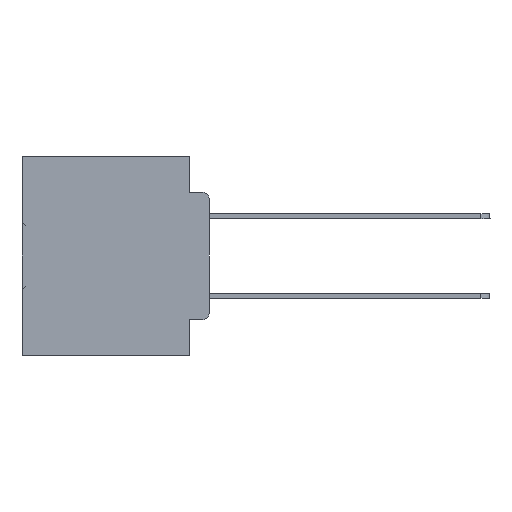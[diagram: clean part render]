
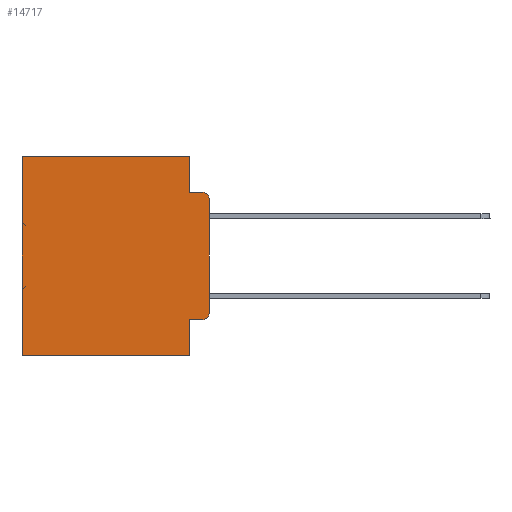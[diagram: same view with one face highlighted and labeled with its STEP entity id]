
A CAD part, left-side view. The second image highlights one B-rep face of the part: STEP entity #14717.
In plain terms, the highlighted planar face has unit normal (-1, 0, 0).
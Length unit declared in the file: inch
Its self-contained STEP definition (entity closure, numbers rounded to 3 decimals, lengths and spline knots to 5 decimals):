
#862 = CARTESIAN_POINT ( 'NONE',  ( 0.298, 0.051, 0. ) ) ;
#1146 = ORIENTED_EDGE ( 'NONE', *, *, #27035, .T. ) ;
#1176 = VERTEX_POINT ( 'NONE', #15526 ) ;
#2767 = DIRECTION ( 'NONE',  ( 0., 1., 0. ) ) ;
#3142 = DIRECTION ( 'NONE',  ( 0., 0., -1. ) ) ;
#3258 = LINE ( 'NONE', #32283, #28905 ) ;
#3944 = DIRECTION ( 'NONE',  ( 0., 1., 0. ) ) ;
#4277 = LINE ( 'NONE', #5706, #37632 ) ;
#4386 = VERTEX_POINT ( 'NONE', #31850 ) ;
#4535 = PLANE ( 'NONE',  #34466 ) ;
#4669 = CARTESIAN_POINT ( 'NONE',  ( 0.298, 0., 0. ) ) ;
#5588 = CARTESIAN_POINT ( 'NONE',  ( 0.298, 0., -0.3915 ) ) ;
#5706 = CARTESIAN_POINT ( 'NONE',  ( 0.298, 0., 0. ) ) ;
#5940 = DIRECTION ( 'NONE',  ( 0., -1., 0. ) ) ;
#7246 = DIRECTION ( 'NONE',  ( 1., 0., 0. ) ) ;
#7446 = VECTOR ( 'NONE', #3944, 39.37008 ) ;
#7640 = DIRECTION ( 'NONE',  ( 0., 0., -1. ) ) ;
#7863 = VERTEX_POINT ( 'NONE', #32480 ) ;
#8265 = DIRECTION ( 'NONE',  ( 0., 0., -1. ) ) ;
#9531 = EDGE_CURVE ( 'NONE', #37716, #35159, #14981, .T. ) ;
#9601 = EDGE_LOOP ( 'NONE', ( #37033, #34493, #10589, #10819, #17951, #32750, #32265, #28895, #12458, #1146 ) ) ;
#10589 = ORIENTED_EDGE ( 'NONE', *, *, #26523, .F. ) ;
#10819 = ORIENTED_EDGE ( 'NONE', *, *, #9531, .F. ) ;
#10880 = AXIS2_PLACEMENT_3D ( 'NONE', #23464, #20653, #3142 ) ;
#11862 = CARTESIAN_POINT ( 'NONE',  ( 0.298, 0.051, -0.0885 ) ) ;
#12153 = EDGE_CURVE ( 'NONE', #37716, #7863, #3258, .T. ) ;
#12458 = ORIENTED_EDGE ( 'NONE', *, *, #17534, .T. ) ;
#12671 = FACE_OUTER_BOUND ( 'NONE', #9601, .T. ) ;
#13833 = VECTOR ( 'NONE', #5940, 39.37008 ) ;
#14717 = ADVANCED_FACE ( 'NONE', ( #12671 ), #4535, .F. ) ;
#14981 = LINE ( 'NONE', #25881, #30955 ) ;
#15052 = CARTESIAN_POINT ( 'NONE',  ( 0.298, 0.051, -0.0885 ) ) ;
#15442 = EDGE_CURVE ( 'NONE', #1176, #4386, #32273, .T. ) ;
#15526 = CARTESIAN_POINT ( 'NONE',  ( 0.298, 0., -0.1085 ) ) ;
#15543 = CIRCLE ( 'NONE', #10880, 0.02 ) ;
#17014 = EDGE_CURVE ( 'NONE', #19408, #22976, #26633, .T. ) ;
#17534 = EDGE_CURVE ( 'NONE', #34117, #25563, #30653, .T. ) ;
#17951 = ORIENTED_EDGE ( 'NONE', *, *, #12153, .T. ) ;
#18342 = EDGE_CURVE ( 'NONE', #34117, #19408, #34751, .T. ) ;
#18680 = VERTEX_POINT ( 'NONE', #5588 ) ;
#18697 = DIRECTION ( 'NONE',  ( 0., 0., -1. ) ) ;
#19233 = CARTESIAN_POINT ( 'NONE',  ( 0.298, 0.051, -0.4115 ) ) ;
#19408 = VERTEX_POINT ( 'NONE', #31348 ) ;
#20653 = DIRECTION ( 'NONE',  ( -1., 0., 0. ) ) ;
#21307 = CARTESIAN_POINT ( 'NONE',  ( 0.298, 0., -0.5 ) ) ;
#21585 = CARTESIAN_POINT ( 'NONE',  ( 0.298, 0.051, -0.4115 ) ) ;
#22516 = LINE ( 'NONE', #31189, #34857 ) ;
#22976 = VERTEX_POINT ( 'NONE', #28055 ) ;
#23464 = CARTESIAN_POINT ( 'NONE',  ( 0.298, 0.02, -0.3915 ) ) ;
#25390 = DIRECTION ( 'NONE',  ( 0., -1., 0. ) ) ;
#25563 = VERTEX_POINT ( 'NONE', #34015 ) ;
#25881 = CARTESIAN_POINT ( 'NONE',  ( 0.298, 0.051, 0. ) ) ;
#26145 = VECTOR ( 'NONE', #25390, 39.37008 ) ;
#26523 = EDGE_CURVE ( 'NONE', #35159, #4386, #37072, .T. ) ;
#26633 = LINE ( 'NONE', #21307, #7446 ) ;
#27035 = EDGE_CURVE ( 'NONE', #25563, #18680, #15543, .T. ) ;
#27625 = AXIS2_PLACEMENT_3D ( 'NONE', #33479, #33345, #36796 ) ;
#28055 = CARTESIAN_POINT ( 'NONE',  ( 0.298, 0.473, -0.5 ) ) ;
#28895 = ORIENTED_EDGE ( 'NONE', *, *, #18342, .F. ) ;
#28905 = VECTOR ( 'NONE', #2767, 39.37008 ) ;
#29671 = VECTOR ( 'NONE', #18697, 39.37008 ) ;
#29848 = DIRECTION ( 'NONE',  ( 0., 0., -1. ) ) ;
#30209 = EDGE_CURVE ( 'NONE', #7863, #22976, #22516, .T. ) ;
#30653 = LINE ( 'NONE', #19233, #26145 ) ;
#30955 = VECTOR ( 'NONE', #8265, 39.37008 ) ;
#31189 = CARTESIAN_POINT ( 'NONE',  ( 0.298, 0.473, 0. ) ) ;
#31348 = CARTESIAN_POINT ( 'NONE',  ( 0.298, 0.051, -0.5 ) ) ;
#31850 = CARTESIAN_POINT ( 'NONE',  ( 0.298, 0.02, -0.0885 ) ) ;
#32265 = ORIENTED_EDGE ( 'NONE', *, *, #17014, .F. ) ;
#32273 = CIRCLE ( 'NONE', #27625, 0.02 ) ;
#32283 = CARTESIAN_POINT ( 'NONE',  ( 0.298, 0., 0. ) ) ;
#32480 = CARTESIAN_POINT ( 'NONE',  ( 0.298, 0.473, 0. ) ) ;
#32750 = ORIENTED_EDGE ( 'NONE', *, *, #30209, .T. ) ;
#33285 = CARTESIAN_POINT ( 'NONE',  ( 0.298, 0.051, 0. ) ) ;
#33345 = DIRECTION ( 'NONE',  ( -1., 0., 0. ) ) ;
#33479 = CARTESIAN_POINT ( 'NONE',  ( 0.298, 0.02, -0.1085 ) ) ;
#34015 = CARTESIAN_POINT ( 'NONE',  ( 0.298, 0.02, -0.4115 ) ) ;
#34117 = VERTEX_POINT ( 'NONE', #21585 ) ;
#34466 = AXIS2_PLACEMENT_3D ( 'NONE', #4669, #7246, #7640 ) ;
#34493 = ORIENTED_EDGE ( 'NONE', *, *, #15442, .T. ) ;
#34518 = DIRECTION ( 'NONE',  ( 0., 0., -1. ) ) ;
#34751 = LINE ( 'NONE', #33285, #29671 ) ;
#34857 = VECTOR ( 'NONE', #34518, 39.37008 ) ;
#35159 = VERTEX_POINT ( 'NONE', #15052 ) ;
#35632 = EDGE_CURVE ( 'NONE', #1176, #18680, #4277, .T. ) ;
#36796 = DIRECTION ( 'NONE',  ( 0., 0., -1. ) ) ;
#37033 = ORIENTED_EDGE ( 'NONE', *, *, #35632, .F. ) ;
#37072 = LINE ( 'NONE', #11862, #13833 ) ;
#37632 = VECTOR ( 'NONE', #29848, 39.37008 ) ;
#37716 = VERTEX_POINT ( 'NONE', #862 ) ;
